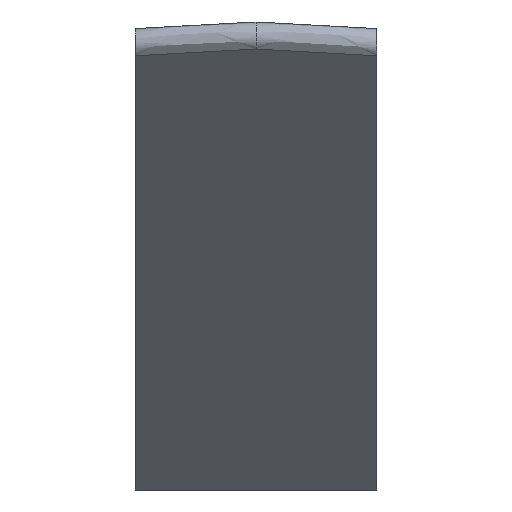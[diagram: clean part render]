
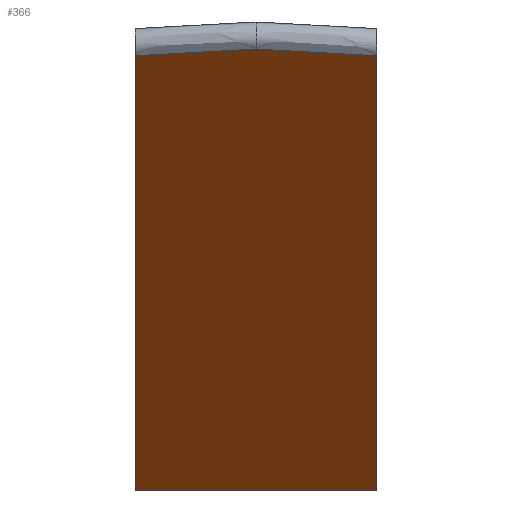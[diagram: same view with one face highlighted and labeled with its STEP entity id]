
A CAD part, top view. The second image highlights one B-rep face of the part: STEP entity #366.
In plain terms, the highlighted planar face has unit normal (0, -0.707, 0.707).
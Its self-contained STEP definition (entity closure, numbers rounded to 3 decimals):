
#16 = VECTOR ( 'NONE', #424, 1000. ) ;
#33 = EDGE_LOOP ( 'NONE', ( #306, #350, #172, #458, #212 ) ) ;
#39 = CARTESIAN_POINT ( 'NONE',  ( -1.898, 1.968, 19.325 ) ) ;
#42 = CARTESIAN_POINT ( 'NONE',  ( 0., 2.073, 19.43 ) ) ;
#64 = CARTESIAN_POINT ( 'NONE',  ( 1.898, -8.678, 8.678 ) ) ;
#65 = VERTEX_POINT ( 'NONE', #175 ) ;
#83 = CARTESIAN_POINT ( 'NONE',  ( -1.898, -4.856, 12.5 ) ) ;
#89 = VECTOR ( 'NONE', #142, 1000. ) ;
#113 = LINE ( 'NONE', #186, #16 ) ;
#116 = VERTEX_POINT ( 'NONE', #272 ) ;
#142 = DIRECTION ( 'NONE',  ( 0., -0.707, -0.707 ) ) ;
#159 = DIRECTION ( 'NONE',  ( 0., 0.707, -0.707 ) ) ;
#160 = CARTESIAN_POINT ( 'NONE',  ( 1.898, -4.856, 12.5 ) ) ;
#162 = VERTEX_POINT ( 'NONE', #404 ) ;
#172 = ORIENTED_EDGE ( 'NONE', *, *, #426, .T. ) ;
#175 = CARTESIAN_POINT ( 'NONE',  ( 0., 2.073, 19.43 ) ) ;
#186 = CARTESIAN_POINT ( 'NONE',  ( -1.898, -8.678, 8.678 ) ) ;
#188 = LINE ( 'NONE', #64, #89 ) ;
#212 = ORIENTED_EDGE ( 'NONE', *, *, #278, .F. ) ;
#221 = CARTESIAN_POINT ( 'NONE',  ( 1.898, 1.968, 19.325 ) ) ;
#230 = EDGE_CURVE ( 'NONE', #162, #65, #376, .T. ) ;
#251 = CARTESIAN_POINT ( 'NONE',  ( -1.268, 2.038, 19.395 ) ) ;
#252 = CARTESIAN_POINT ( 'NONE',  ( 0.634, 2.073, 19.43 ) ) ;
#272 = CARTESIAN_POINT ( 'NONE',  ( -1.898, 1.968, 19.325 ) ) ;
#278 = EDGE_CURVE ( 'NONE', #328, #453, #386, .T. ) ;
#280 = CARTESIAN_POINT ( 'NONE',  ( 1.898, -4.856, 12.5 ) ) ;
#298 = PLANE ( 'NONE',  #480 ) ;
#305 = EDGE_CURVE ( 'NONE', #116, #453, #113, .T. ) ;
#306 = ORIENTED_EDGE ( 'NONE', *, *, #330, .F. ) ;
#313 = VECTOR ( 'NONE', #448, 1000. ) ;
#328 = VERTEX_POINT ( 'NONE', #280 ) ;
#330 = EDGE_CURVE ( 'NONE', #162, #328, #188, .T. ) ;
#348 =( BOUNDED_CURVE ( )  B_SPLINE_CURVE ( 3, ( #413, #479, #251, #39 ),
 .UNSPECIFIED., .F., .F. ) 
 B_SPLINE_CURVE_WITH_KNOTS ( ( 4, 4 ),
 ( 0., 0.11 ),
 .UNSPECIFIED. ) 
 CURVE ( )  GEOMETRIC_REPRESENTATION_ITEM ( )  RATIONAL_B_SPLINE_CURVE ( ( 1., 0.999, 0.999, 1. ) ) 
 REPRESENTATION_ITEM ( '' )  );
#350 = ORIENTED_EDGE ( 'NONE', *, *, #230, .T. ) ;
#366 = ADVANCED_FACE ( 'NONE', ( #384 ), #298, .F. ) ;
#376 =( BOUNDED_CURVE ( )  B_SPLINE_CURVE ( 3, ( #221, #446, #252, #42 ),
 .UNSPECIFIED., .F., .F. ) 
 B_SPLINE_CURVE_WITH_KNOTS ( ( 4, 4 ),
 ( 6.173, 6.283 ),
 .UNSPECIFIED. ) 
 CURVE ( )  GEOMETRIC_REPRESENTATION_ITEM ( )  RATIONAL_B_SPLINE_CURVE ( ( 1., 0.999, 0.999, 1. ) ) 
 REPRESENTATION_ITEM ( '' )  );
#384 = FACE_OUTER_BOUND ( 'NONE', #33, .T. ) ;
#386 = LINE ( 'NONE', #160, #313 ) ;
#391 = CARTESIAN_POINT ( 'NONE',  ( 1.898, -8.678, 8.678 ) ) ;
#404 = CARTESIAN_POINT ( 'NONE',  ( 1.898, 1.968, 19.325 ) ) ;
#413 = CARTESIAN_POINT ( 'NONE',  ( 0., 2.073, 19.43 ) ) ;
#424 = DIRECTION ( 'NONE',  ( 0., -0.707, -0.707 ) ) ;
#425 = DIRECTION ( 'NONE',  ( 0., 0.707, 0.707 ) ) ;
#426 = EDGE_CURVE ( 'NONE', #65, #116, #348, .T. ) ;
#446 = CARTESIAN_POINT ( 'NONE',  ( 1.268, 2.038, 19.395 ) ) ;
#448 = DIRECTION ( 'NONE',  ( -1., 0., 0. ) ) ;
#453 = VERTEX_POINT ( 'NONE', #83 ) ;
#458 = ORIENTED_EDGE ( 'NONE', *, *, #305, .T. ) ;
#479 = CARTESIAN_POINT ( 'NONE',  ( -0.634, 2.073, 19.43 ) ) ;
#480 = AXIS2_PLACEMENT_3D ( 'NONE', #391, #159, #425 ) ;
